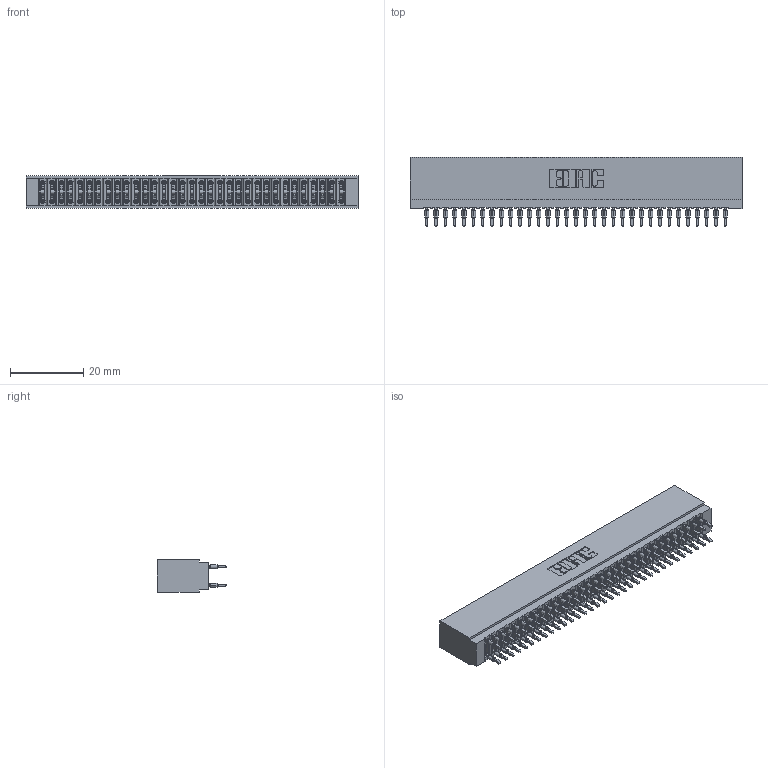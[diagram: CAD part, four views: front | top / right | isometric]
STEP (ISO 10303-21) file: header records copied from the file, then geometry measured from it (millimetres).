
FILE_DESCRIPTION (( 'STEP AP203' ), '1' );
FILE_NAME ('725-066-560-201.STEP', '2026-02-24T18:28:45', ( '' ), ( '' ), 'SwSTEP 2.0', 'SolidWorks 2023', '' );
FILE_SCHEMA (( 'CONFIG_CONTROL_DESIGN' ));
Length unit declared in the file: millimetre
Products named in the file (3): 725-066-560-201; 745-292-001_560; 725 Part_Insulator Option - 01
Assembly tree (67 placements, depth 2):
  725-066-560-201
    725 Part_Insulator Option - 01
    745-292-001_560  x66
Bounding box: 90.42 x 18.8 x 8.89 mm (x, y, z)
Volume: 7459.9 mm3; surface area: 16604.3 mm2
Topology: 67 solids, 67 shells, 6596 faces, 18041 edges, 11454 vertices
Faces by surface type: plane 3421, cylinder 1459, bspline 1320, torus 396
Entity records: 57072 total; most frequent: CARTESIAN_POINT 10405, ORIENTED_EDGE 9822, DIRECTION 8595, EDGE_CURVE 4911, VECTOR 4523, LINE 4523, VERTEX_POINT 3134, AXIS2_PLACEMENT_3D 2036
